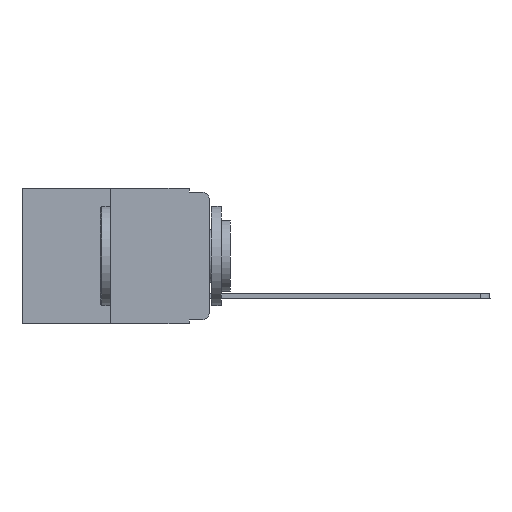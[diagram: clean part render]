
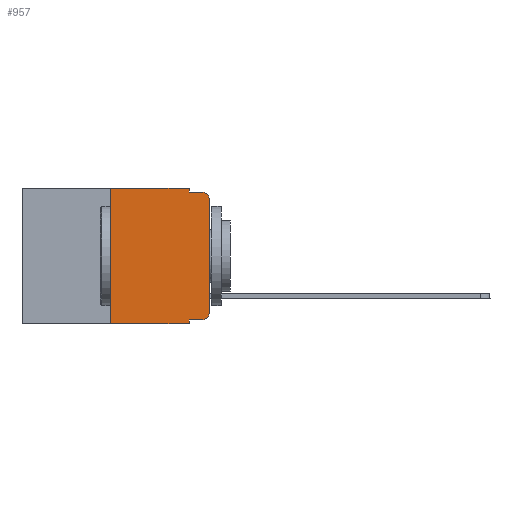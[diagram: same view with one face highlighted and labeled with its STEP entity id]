
A CAD part, left-side view. The second image highlights one B-rep face of the part: STEP entity #957.
In plain terms, the highlighted planar face has unit normal (-1, 0, 0).
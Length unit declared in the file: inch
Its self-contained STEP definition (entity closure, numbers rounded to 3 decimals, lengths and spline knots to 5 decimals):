
#321 = LINE ( 'NONE', #5759, #4546 ) ;
#376 = DIRECTION ( 'NONE',  ( 1., 0., 0. ) ) ;
#464 = VERTEX_POINT ( 'NONE', #3683 ) ;
#957 = ADVANCED_FACE ( 'NONE', ( #8975 ), #11042, .F. ) ;
#1190 = CARTESIAN_POINT ( 'NONE',  ( 0., 0.02, -0.01 ) ) ;
#1804 = CIRCLE ( 'NONE', #8043, 0.02 ) ;
#1952 = CARTESIAN_POINT ( 'NONE',  ( 0., 0.473, -0.343 ) ) ;
#2166 = VERTEX_POINT ( 'NONE', #15774 ) ;
#2184 = LINE ( 'NONE', #3656, #11960 ) ;
#2344 = DIRECTION ( 'NONE',  ( 0., -1., 0. ) ) ;
#3596 = CARTESIAN_POINT ( 'NONE',  ( 0., 0.051, 0. ) ) ;
#3656 = CARTESIAN_POINT ( 'NONE',  ( 0., 0., 0. ) ) ;
#3683 = CARTESIAN_POINT ( 'NONE',  ( 0., 0.051, -0.01 ) ) ;
#3692 = CIRCLE ( 'NONE', #22479, 0.02 ) ;
#4546 = VECTOR ( 'NONE', #2344, 39.37008 ) ;
#4696 = EDGE_CURVE ( 'NONE', #2166, #15966, #2184, .T. ) ;
#5106 = EDGE_CURVE ( 'NONE', #10017, #18338, #21398, .T. ) ;
#5559 = LINE ( 'NONE', #22730, #19801 ) ;
#5759 = CARTESIAN_POINT ( 'NONE',  ( 0., 0.051, -0.333 ) ) ;
#5772 = VERTEX_POINT ( 'NONE', #21242 ) ;
#6091 = CARTESIAN_POINT ( 'NONE',  ( 0., 0.02, -0.03 ) ) ;
#6833 = LINE ( 'NONE', #12876, #12394 ) ;
#7030 = CARTESIAN_POINT ( 'NONE',  ( 0., 0.051, -0.333 ) ) ;
#7671 = ORIENTED_EDGE ( 'NONE', *, *, #5106, .F. ) ;
#8043 = AXIS2_PLACEMENT_3D ( 'NONE', #14779, #11077, #9066 ) ;
#8077 = EDGE_CURVE ( 'NONE', #10017, #14542, #321, .T. ) ;
#8184 = EDGE_CURVE ( 'NONE', #15966, #22728, #3692, .T. ) ;
#8339 = VECTOR ( 'NONE', #16073, 39.37008 ) ;
#8975 = FACE_OUTER_BOUND ( 'NONE', #22315, .T. ) ;
#9065 = ORIENTED_EDGE ( 'NONE', *, *, #4696, .T. ) ;
#9066 = DIRECTION ( 'NONE',  ( 0., 0., -1. ) ) ;
#9425 = ORIENTED_EDGE ( 'NONE', *, *, #17764, .F. ) ;
#10017 = VERTEX_POINT ( 'NONE', #7030 ) ;
#10133 = VECTOR ( 'NONE', #16239, 39.37008 ) ;
#10291 = CARTESIAN_POINT ( 'NONE',  ( 0., 0.02, -0.333 ) ) ;
#10784 = VERTEX_POINT ( 'NONE', #21776 ) ;
#10941 = DIRECTION ( 'NONE',  ( 0., 0., -1. ) ) ;
#11042 = PLANE ( 'NONE',  #20112 ) ;
#11077 = DIRECTION ( 'NONE',  ( -1., 0., 0. ) ) ;
#11366 = DIRECTION ( 'NONE',  ( -1., 0., 0. ) ) ;
#11656 = EDGE_CURVE ( 'NONE', #10784, #17331, #19456, .T. ) ;
#11960 = VECTOR ( 'NONE', #21641, 39.37008 ) ;
#12394 = VECTOR ( 'NONE', #21826, 39.37008 ) ;
#12713 = EDGE_CURVE ( 'NONE', #14542, #2166, #1804, .T. ) ;
#12876 = CARTESIAN_POINT ( 'NONE',  ( 0., 0.051, -0.01 ) ) ;
#13594 = VECTOR ( 'NONE', #17747, 39.37008 ) ;
#13730 = CARTESIAN_POINT ( 'NONE',  ( 0., 0., -0.03 ) ) ;
#14542 = VERTEX_POINT ( 'NONE', #10291 ) ;
#14779 = CARTESIAN_POINT ( 'NONE',  ( 0., 0.02, -0.313 ) ) ;
#14982 = VECTOR ( 'NONE', #10941, 39.37008 ) ;
#15051 = CARTESIAN_POINT ( 'NONE',  ( 0., 0.25, 0. ) ) ;
#15426 = ORIENTED_EDGE ( 'NONE', *, *, #12713, .T. ) ;
#15725 = EDGE_CURVE ( 'NONE', #17331, #5772, #5559, .T. ) ;
#15774 = CARTESIAN_POINT ( 'NONE',  ( 0., 0., -0.313 ) ) ;
#15869 = CARTESIAN_POINT ( 'NONE',  ( 0., 0.051, -0.343 ) ) ;
#15880 = ORIENTED_EDGE ( 'NONE', *, *, #22693, .T. ) ;
#15934 = CARTESIAN_POINT ( 'NONE',  ( 0., 0.25, 0. ) ) ;
#15966 = VERTEX_POINT ( 'NONE', #13730 ) ;
#16073 = DIRECTION ( 'NONE',  ( 0., 0., -1. ) ) ;
#16239 = DIRECTION ( 'NONE',  ( 0., -1., 0. ) ) ;
#16265 = CARTESIAN_POINT ( 'NONE',  ( 0., 0.051, 0. ) ) ;
#17300 = DIRECTION ( 'NONE',  ( 0., -1., 0. ) ) ;
#17331 = VERTEX_POINT ( 'NONE', #15051 ) ;
#17747 = DIRECTION ( 'NONE',  ( 0., 0., 1. ) ) ;
#17764 = EDGE_CURVE ( 'NONE', #5772, #464, #23034, .T. ) ;
#17886 = ORIENTED_EDGE ( 'NONE', *, *, #18496, .F. ) ;
#17980 = ORIENTED_EDGE ( 'NONE', *, *, #15725, .F. ) ;
#18338 = VERTEX_POINT ( 'NONE', #15869 ) ;
#18496 = EDGE_CURVE ( 'NONE', #464, #22728, #6833, .T. ) ;
#18741 = DIRECTION ( 'NONE',  ( 0., 0., -1. ) ) ;
#19456 = LINE ( 'NONE', #15934, #13594 ) ;
#19801 = VECTOR ( 'NONE', #17300, 39.37008 ) ;
#19849 = LINE ( 'NONE', #1952, #10133 ) ;
#20112 = AXIS2_PLACEMENT_3D ( 'NONE', #20597, #376, #20445 ) ;
#20445 = DIRECTION ( 'NONE',  ( 0., 0., -1. ) ) ;
#20597 = CARTESIAN_POINT ( 'NONE',  ( 0., 0.473, 0. ) ) ;
#20608 = ORIENTED_EDGE ( 'NONE', *, *, #8184, .T. ) ;
#20903 = ORIENTED_EDGE ( 'NONE', *, *, #11656, .F. ) ;
#21242 = CARTESIAN_POINT ( 'NONE',  ( 0., 0.051, 0. ) ) ;
#21398 = LINE ( 'NONE', #3596, #8339 ) ;
#21641 = DIRECTION ( 'NONE',  ( 0., 0., 1. ) ) ;
#21776 = CARTESIAN_POINT ( 'NONE',  ( 0., 0.25, -0.343 ) ) ;
#21826 = DIRECTION ( 'NONE',  ( 0., -1., 0. ) ) ;
#22222 = ORIENTED_EDGE ( 'NONE', *, *, #8077, .T. ) ;
#22315 = EDGE_LOOP ( 'NONE', ( #9065, #20608, #17886, #9425, #17980, #20903, #15880, #7671, #22222, #15426 ) ) ;
#22479 = AXIS2_PLACEMENT_3D ( 'NONE', #6091, #11366, #18741 ) ;
#22693 = EDGE_CURVE ( 'NONE', #10784, #18338, #19849, .T. ) ;
#22728 = VERTEX_POINT ( 'NONE', #1190 ) ;
#22730 = CARTESIAN_POINT ( 'NONE',  ( 0., 0.473, 0. ) ) ;
#23034 = LINE ( 'NONE', #16265, #14982 ) ;
